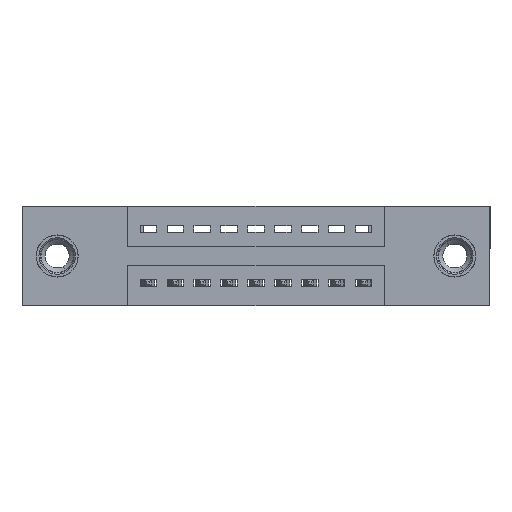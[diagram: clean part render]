
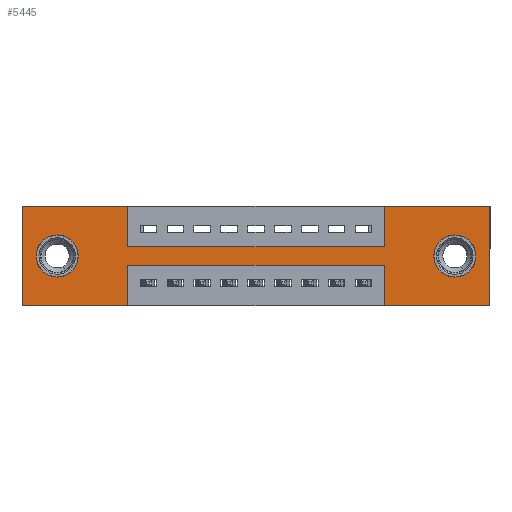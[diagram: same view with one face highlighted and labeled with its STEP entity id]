
A CAD part, front view. The second image highlights one B-rep face of the part: STEP entity #5445.
In plain terms, the highlighted planar face has unit normal (0, -1, 0).
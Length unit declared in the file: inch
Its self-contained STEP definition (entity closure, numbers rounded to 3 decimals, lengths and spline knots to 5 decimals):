
#46 = CARTESIAN_POINT ( 'NONE',  ( 0.3925, 0., -0.37 ) ) ;
#54 = LINE ( 'NONE', #11198, #10562 ) ;
#55 = DIRECTION ( 'NONE',  ( 1., 0., 0. ) ) ;
#148 = VERTEX_POINT ( 'NONE', #11675 ) ;
#189 = DIRECTION ( 'NONE',  ( 0., 0., -1. ) ) ;
#248 = CIRCLE ( 'NONE', #9173, 0.078 ) ;
#479 = ORIENTED_EDGE ( 'NONE', *, *, #9488, .F. ) ;
#739 = CARTESIAN_POINT ( 'NONE',  ( 1.735, 0., 0. ) ) ;
#981 = LINE ( 'NONE', #10668, #1134 ) ;
#1008 = DIRECTION ( 'NONE',  ( 0., 1., 0. ) ) ;
#1118 = CARTESIAN_POINT ( 'NONE',  ( 0.3925, 0., -0.15 ) ) ;
#1134 = VECTOR ( 'NONE', #189, 39.37008 ) ;
#1148 = DIRECTION ( 'NONE',  ( 1., 0., 0. ) ) ;
#1242 = LINE ( 'NONE', #6857, #6398 ) ;
#1282 = EDGE_LOOP ( 'NONE', ( #7404, #12109 ) ) ;
#1407 = LINE ( 'NONE', #3209, #13231 ) ;
#1430 = CARTESIAN_POINT ( 'NONE',  ( 1.605, 0., -0.263 ) ) ;
#1591 = DIRECTION ( 'NONE',  ( 0., 0., -1. ) ) ;
#1633 = AXIS2_PLACEMENT_3D ( 'NONE', #4879, #12085, #8945 ) ;
#1664 = FACE_BOUND ( 'NONE', #1282, .T. ) ;
#1913 = EDGE_LOOP ( 'NONE', ( #479, #10766, #4324, #2738, #11954, #7328, #8666, #3646, #3955, #9709, #8375, #8734 ) ) ;
#1980 = FACE_BOUND ( 'NONE', #12651, .T. ) ;
#1987 = VERTEX_POINT ( 'NONE', #10683 ) ;
#2233 = EDGE_CURVE ( 'NONE', #3789, #3918, #248, .T. ) ;
#2522 = LINE ( 'NONE', #11649, #13200 ) ;
#2672 = CARTESIAN_POINT ( 'NONE',  ( 0.13, 0., -0.185 ) ) ;
#2738 = ORIENTED_EDGE ( 'NONE', *, *, #11295, .F. ) ;
#2753 = CARTESIAN_POINT ( 'NONE',  ( 0., 0., 0. ) ) ;
#2837 = VECTOR ( 'NONE', #55, 39.37008 ) ;
#2882 = VERTEX_POINT ( 'NONE', #46 ) ;
#2929 = DIRECTION ( 'NONE',  ( 0., 0., 1. ) ) ;
#3183 = EDGE_CURVE ( 'NONE', #148, #1987, #9806, .T. ) ;
#3209 = CARTESIAN_POINT ( 'NONE',  ( 0.3925, 0., -0.15 ) ) ;
#3217 = DIRECTION ( 'NONE',  ( -1., 0., 0. ) ) ;
#3327 = LINE ( 'NONE', #8082, #2837 ) ;
#3359 = LINE ( 'NONE', #12947, #4642 ) ;
#3646 = ORIENTED_EDGE ( 'NONE', *, *, #12175, .F. ) ;
#3789 = VERTEX_POINT ( 'NONE', #1430 ) ;
#3804 = DIRECTION ( 'NONE',  ( 0., 0., 1. ) ) ;
#3918 = VERTEX_POINT ( 'NONE', #4075 ) ;
#3940 = VERTEX_POINT ( 'NONE', #10243 ) ;
#3955 = ORIENTED_EDGE ( 'NONE', *, *, #13273, .F. ) ;
#4075 = CARTESIAN_POINT ( 'NONE',  ( 1.605, 0., -0.107 ) ) ;
#4099 = VECTOR ( 'NONE', #9731, 39.37008 ) ;
#4171 = VECTOR ( 'NONE', #3217, 39.37008 ) ;
#4302 = DIRECTION ( 'NONE',  ( 0., 0., -1. ) ) ;
#4324 = ORIENTED_EDGE ( 'NONE', *, *, #5384, .F. ) ;
#4606 = VECTOR ( 'NONE', #10907, 39.37008 ) ;
#4615 = EDGE_CURVE ( 'NONE', #12376, #8275, #10584, .T. ) ;
#4642 = VECTOR ( 'NONE', #12529, 39.37008 ) ;
#4706 = CIRCLE ( 'NONE', #6486, 0.078 ) ;
#4725 = DIRECTION ( 'NONE',  ( 0., 1., 0. ) ) ;
#4809 = CARTESIAN_POINT ( 'NONE',  ( 0.3925, 0., -0.22 ) ) ;
#4853 = EDGE_CURVE ( 'NONE', #3918, #3789, #8444, .T. ) ;
#4879 = CARTESIAN_POINT ( 'NONE',  ( 0., 0., -0.37 ) ) ;
#5067 = CARTESIAN_POINT ( 'NONE',  ( 0., 0., -0.37 ) ) ;
#5243 = VERTEX_POINT ( 'NONE', #9512 ) ;
#5384 = EDGE_CURVE ( 'NONE', #6199, #148, #54, .T. ) ;
#5445 = ADVANCED_FACE ( 'NONE', ( #1664, #1980, #11395 ), #11048, .T. ) ;
#5809 = LINE ( 'NONE', #6429, #7581 ) ;
#6094 = DIRECTION ( 'NONE',  ( 0., 0., -1. ) ) ;
#6166 = CARTESIAN_POINT ( 'NONE',  ( 0., 0., -0.37 ) ) ;
#6199 = VERTEX_POINT ( 'NONE', #12180 ) ;
#6307 = VERTEX_POINT ( 'NONE', #7080 ) ;
#6398 = VECTOR ( 'NONE', #1591, 39.37008 ) ;
#6429 = CARTESIAN_POINT ( 'NONE',  ( 0., 0., 0. ) ) ;
#6452 = CIRCLE ( 'NONE', #12943, 0.078 ) ;
#6486 = AXIS2_PLACEMENT_3D ( 'NONE', #13197, #6970, #2929 ) ;
#6689 = CARTESIAN_POINT ( 'NONE',  ( 1.3425, 0., 0. ) ) ;
#6755 = DIRECTION ( 'NONE',  ( 0., 1., 0. ) ) ;
#6857 = CARTESIAN_POINT ( 'NONE',  ( 1.735, 0., 0. ) ) ;
#6970 = DIRECTION ( 'NONE',  ( 0., 1., 0. ) ) ;
#7067 = VERTEX_POINT ( 'NONE', #1118 ) ;
#7080 = CARTESIAN_POINT ( 'NONE',  ( 0., 0., -0.37 ) ) ;
#7328 = ORIENTED_EDGE ( 'NONE', *, *, #13185, .F. ) ;
#7404 = ORIENTED_EDGE ( 'NONE', *, *, #4853, .T. ) ;
#7581 = VECTOR ( 'NONE', #10530, 39.37008 ) ;
#7583 = VERTEX_POINT ( 'NONE', #739 ) ;
#7671 = LINE ( 'NONE', #5067, #11416 ) ;
#7903 = CARTESIAN_POINT ( 'NONE',  ( 1.605, 0., -0.185 ) ) ;
#8082 = CARTESIAN_POINT ( 'NONE',  ( 0., 0., 0. ) ) ;
#8275 = VERTEX_POINT ( 'NONE', #12591 ) ;
#8366 = CARTESIAN_POINT ( 'NONE',  ( 0.13, 0., -0.263 ) ) ;
#8375 = ORIENTED_EDGE ( 'NONE', *, *, #10904, .F. ) ;
#8444 = CIRCLE ( 'NONE', #13379, 0.078 ) ;
#8561 = EDGE_CURVE ( 'NONE', #12091, #5243, #3359, .T. ) ;
#8666 = ORIENTED_EDGE ( 'NONE', *, *, #4615, .F. ) ;
#8734 = ORIENTED_EDGE ( 'NONE', *, *, #9192, .F. ) ;
#8945 = DIRECTION ( 'NONE',  ( 0., 0., -1. ) ) ;
#9081 = DIRECTION ( 'NONE',  ( -1., 0., 0. ) ) ;
#9085 = CARTESIAN_POINT ( 'NONE',  ( 1.605, 0., -0.185 ) ) ;
#9173 = AXIS2_PLACEMENT_3D ( 'NONE', #9085, #1008, #6094 ) ;
#9192 = EDGE_CURVE ( 'NONE', #2882, #6307, #7671, .T. ) ;
#9306 = ORIENTED_EDGE ( 'NONE', *, *, #9594, .T. ) ;
#9488 = EDGE_CURVE ( 'NONE', #1987, #2882, #981, .T. ) ;
#9512 = CARTESIAN_POINT ( 'NONE',  ( 0.3925, 0., 0. ) ) ;
#9594 = EDGE_CURVE ( 'NONE', #11693, #9714, #6452, .T. ) ;
#9709 = ORIENTED_EDGE ( 'NONE', *, *, #8561, .F. ) ;
#9714 = VERTEX_POINT ( 'NONE', #13063 ) ;
#9731 = DIRECTION ( 'NONE',  ( 0., 0., 1. ) ) ;
#9806 = LINE ( 'NONE', #4809, #4606 ) ;
#9821 = EDGE_CURVE ( 'NONE', #9714, #11693, #4706, .T. ) ;
#10243 = CARTESIAN_POINT ( 'NONE',  ( 1.735, 0., -0.37 ) ) ;
#10262 = CARTESIAN_POINT ( 'NONE',  ( 1.3425, 0., -0.15 ) ) ;
#10530 = DIRECTION ( 'NONE',  ( 0., 0., 1. ) ) ;
#10562 = VECTOR ( 'NONE', #3804, 39.37008 ) ;
#10584 = LINE ( 'NONE', #6689, #4099 ) ;
#10668 = CARTESIAN_POINT ( 'NONE',  ( 0.3925, 0., -0.37 ) ) ;
#10683 = CARTESIAN_POINT ( 'NONE',  ( 0.3925, 0., -0.22 ) ) ;
#10766 = ORIENTED_EDGE ( 'NONE', *, *, #3183, .F. ) ;
#10904 = EDGE_CURVE ( 'NONE', #6307, #12091, #5809, .T. ) ;
#10907 = DIRECTION ( 'NONE',  ( -1., 0., 0. ) ) ;
#11048 = PLANE ( 'NONE',  #1633 ) ;
#11198 = CARTESIAN_POINT ( 'NONE',  ( 1.3425, 0., -0.37 ) ) ;
#11295 = EDGE_CURVE ( 'NONE', #3940, #6199, #13091, .T. ) ;
#11395 = FACE_OUTER_BOUND ( 'NONE', #1913, .T. ) ;
#11416 = VECTOR ( 'NONE', #9081, 39.37008 ) ;
#11649 = CARTESIAN_POINT ( 'NONE',  ( 0.3925, 0., 0. ) ) ;
#11675 = CARTESIAN_POINT ( 'NONE',  ( 1.3425, 0., -0.22 ) ) ;
#11693 = VERTEX_POINT ( 'NONE', #8366 ) ;
#11807 = EDGE_CURVE ( 'NONE', #7583, #3940, #1242, .T. ) ;
#11853 = ORIENTED_EDGE ( 'NONE', *, *, #9821, .T. ) ;
#11945 = DIRECTION ( 'NONE',  ( 0., 0., 1. ) ) ;
#11954 = ORIENTED_EDGE ( 'NONE', *, *, #11807, .F. ) ;
#12085 = DIRECTION ( 'NONE',  ( 0., -1., 0. ) ) ;
#12091 = VERTEX_POINT ( 'NONE', #2753 ) ;
#12109 = ORIENTED_EDGE ( 'NONE', *, *, #2233, .T. ) ;
#12175 = EDGE_CURVE ( 'NONE', #7067, #12376, #1407, .T. ) ;
#12180 = CARTESIAN_POINT ( 'NONE',  ( 1.3425, 0., -0.37 ) ) ;
#12376 = VERTEX_POINT ( 'NONE', #10262 ) ;
#12529 = DIRECTION ( 'NONE',  ( 1., 0., 0. ) ) ;
#12591 = CARTESIAN_POINT ( 'NONE',  ( 1.3425, 0., 0. ) ) ;
#12651 = EDGE_LOOP ( 'NONE', ( #11853, #9306 ) ) ;
#12943 = AXIS2_PLACEMENT_3D ( 'NONE', #2672, #4725, #11945 ) ;
#12947 = CARTESIAN_POINT ( 'NONE',  ( 0., 0., 0. ) ) ;
#13063 = CARTESIAN_POINT ( 'NONE',  ( 0.13, 0., -0.107 ) ) ;
#13091 = LINE ( 'NONE', #6166, #4171 ) ;
#13135 = DIRECTION ( 'NONE',  ( 0., 0., -1. ) ) ;
#13185 = EDGE_CURVE ( 'NONE', #8275, #7583, #3327, .T. ) ;
#13197 = CARTESIAN_POINT ( 'NONE',  ( 0.13, 0., -0.185 ) ) ;
#13200 = VECTOR ( 'NONE', #4302, 39.37008 ) ;
#13231 = VECTOR ( 'NONE', #1148, 39.37008 ) ;
#13273 = EDGE_CURVE ( 'NONE', #5243, #7067, #2522, .T. ) ;
#13379 = AXIS2_PLACEMENT_3D ( 'NONE', #7903, #6755, #13135 ) ;
